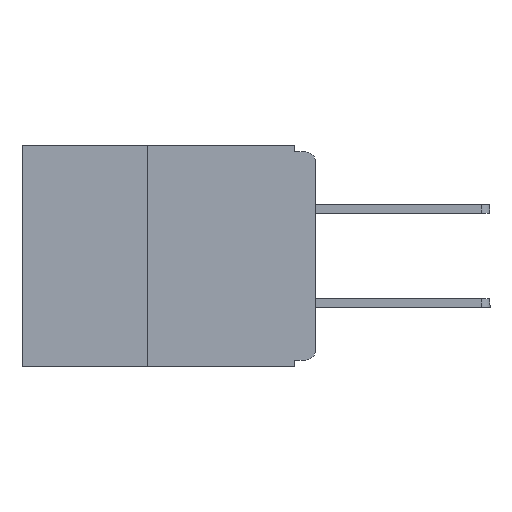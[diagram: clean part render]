
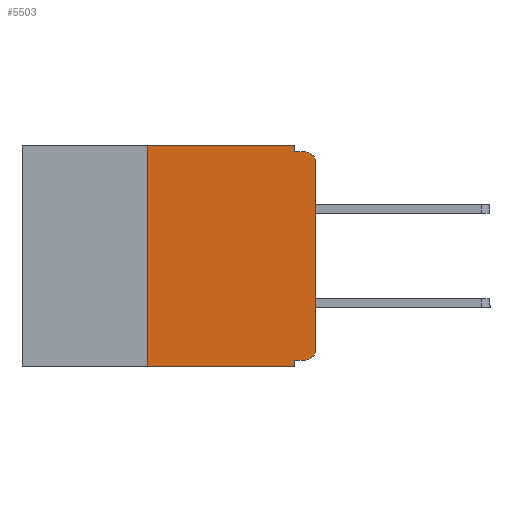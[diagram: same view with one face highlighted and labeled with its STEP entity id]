
A CAD part, left-side view. The second image highlights one B-rep face of the part: STEP entity #5503.
In plain terms, the highlighted planar face has unit normal (-1, 0, 0).
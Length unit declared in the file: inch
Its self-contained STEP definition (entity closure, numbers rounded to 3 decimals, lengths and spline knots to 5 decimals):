
#1129 = CARTESIAN_POINT ( 'NONE',  ( 0., 0.015, -0.01 ) ) ;
#1222 = CARTESIAN_POINT ( 'NONE',  ( 0., 0.25, 0. ) ) ;
#1565 = AXIS2_PLACEMENT_3D ( 'NONE', #5508, #13372, #6719 ) ;
#1937 = DIRECTION ( 'NONE',  ( 0., 0., 1. ) ) ;
#1966 = DIRECTION ( 'NONE',  ( 0., 0., -1. ) ) ;
#1986 = DIRECTION ( 'NONE',  ( 1., 0., 0. ) ) ;
#2007 = PLANE ( 'NONE',  #13067 ) ;
#2136 = CARTESIAN_POINT ( 'NONE',  ( 0., 0., -0.01 ) ) ;
#2154 = CARTESIAN_POINT ( 'NONE',  ( 0., 0.437, 0. ) ) ;
#2473 = FACE_OUTER_BOUND ( 'NONE', #12081, .T. ) ;
#2479 = VECTOR ( 'NONE', #6646, 39.37008 ) ;
#2536 = ORIENTED_EDGE ( 'NONE', *, *, #13126, .T. ) ;
#2957 = CARTESIAN_POINT ( 'NONE',  ( 0., 0., 0. ) ) ;
#3053 = LINE ( 'NONE', #10848, #14313 ) ;
#3094 = ORIENTED_EDGE ( 'NONE', *, *, #9424, .T. ) ;
#3125 = ORIENTED_EDGE ( 'NONE', *, *, #6260, .F. ) ;
#3194 = EDGE_CURVE ( 'NONE', #7947, #13280, #8759, .T. ) ;
#3290 = DIRECTION ( 'NONE',  ( 0., -1., 0. ) ) ;
#3303 = ORIENTED_EDGE ( 'NONE', *, *, #8119, .T. ) ;
#3767 = CARTESIAN_POINT ( 'NONE',  ( 0., 0.25, -0.33 ) ) ;
#4493 = VERTEX_POINT ( 'NONE', #13315 ) ;
#4528 = LINE ( 'NONE', #5465, #4894 ) ;
#4581 = VERTEX_POINT ( 'NONE', #12604 ) ;
#4690 = ORIENTED_EDGE ( 'NONE', *, *, #8791, .F. ) ;
#4702 = VECTOR ( 'NONE', #6702, 39.37008 ) ;
#4733 = ORIENTED_EDGE ( 'NONE', *, *, #3194, .F. ) ;
#4763 = CARTESIAN_POINT ( 'NONE',  ( 0., 0.031, 0. ) ) ;
#4802 = CARTESIAN_POINT ( 'NONE',  ( 0., 0., -0.025 ) ) ;
#4886 = VERTEX_POINT ( 'NONE', #9381 ) ;
#4894 = VECTOR ( 'NONE', #14404, 39.37008 ) ;
#5351 = VERTEX_POINT ( 'NONE', #4802 ) ;
#5465 = CARTESIAN_POINT ( 'NONE',  ( 0., 0.437, 0. ) ) ;
#5503 = ADVANCED_FACE ( 'NONE', ( #2473 ), #2007, .F. ) ;
#5508 = CARTESIAN_POINT ( 'NONE',  ( 0., 0.015, -0.305 ) ) ;
#5520 = LINE ( 'NONE', #13312, #2479 ) ;
#5572 = ORIENTED_EDGE ( 'NONE', *, *, #12054, .F. ) ;
#5578 = VECTOR ( 'NONE', #1937, 39.37008 ) ;
#5779 = VERTEX_POINT ( 'NONE', #1129 ) ;
#6260 = EDGE_CURVE ( 'NONE', #4581, #7574, #5520, .T. ) ;
#6646 = DIRECTION ( 'NONE',  ( 0., 0., -1. ) ) ;
#6651 = CARTESIAN_POINT ( 'NONE',  ( 0., 0.015, -0.025 ) ) ;
#6702 = DIRECTION ( 'NONE',  ( 0., -1., 0. ) ) ;
#6719 = DIRECTION ( 'NONE',  ( 0., 0., -1. ) ) ;
#7454 = EDGE_CURVE ( 'NONE', #4493, #5351, #14241, .T. ) ;
#7574 = VERTEX_POINT ( 'NONE', #11229 ) ;
#7851 = LINE ( 'NONE', #11214, #4702 ) ;
#7855 = DIRECTION ( 'NONE',  ( 0., 0., -1. ) ) ;
#7947 = VERTEX_POINT ( 'NONE', #3767 ) ;
#8119 = EDGE_CURVE ( 'NONE', #5351, #5779, #13058, .T. ) ;
#8693 = CARTESIAN_POINT ( 'NONE',  ( 0., 0.031, -0.01 ) ) ;
#8759 = LINE ( 'NONE', #14010, #5578 ) ;
#8783 = CIRCLE ( 'NONE', #1565, 0.015 ) ;
#8791 = EDGE_CURVE ( 'NONE', #13280, #14341, #4528, .T. ) ;
#8995 = LINE ( 'NONE', #2136, #14379 ) ;
#9381 = CARTESIAN_POINT ( 'NONE',  ( 0., 0.015, -0.32 ) ) ;
#9424 = EDGE_CURVE ( 'NONE', #7947, #7574, #7851, .T. ) ;
#9477 = DIRECTION ( 'NONE',  ( 0., 0., -1. ) ) ;
#10304 = EDGE_CURVE ( 'NONE', #14341, #10970, #13990, .T. ) ;
#10848 = CARTESIAN_POINT ( 'NONE',  ( 0., 0., -0.32 ) ) ;
#10970 = VERTEX_POINT ( 'NONE', #8693 ) ;
#11214 = CARTESIAN_POINT ( 'NONE',  ( 0., 0.437, -0.33 ) ) ;
#11229 = CARTESIAN_POINT ( 'NONE',  ( 0., 0.031, -0.33 ) ) ;
#11379 = AXIS2_PLACEMENT_3D ( 'NONE', #6651, #14397, #7855 ) ;
#11402 = VECTOR ( 'NONE', #12088, 39.37008 ) ;
#11905 = DIRECTION ( 'NONE',  ( 0., 1., 0. ) ) ;
#12054 = EDGE_CURVE ( 'NONE', #10970, #5779, #8995, .T. ) ;
#12081 = EDGE_LOOP ( 'NONE', ( #13181, #3303, #5572, #13323, #4690, #4733, #3094, #3125, #12618, #2536 ) ) ;
#12088 = DIRECTION ( 'NONE',  ( 0., 0., 1. ) ) ;
#12564 = CARTESIAN_POINT ( 'NONE',  ( 0., 0.031, 0. ) ) ;
#12604 = CARTESIAN_POINT ( 'NONE',  ( 0., 0.031, -0.32 ) ) ;
#12618 = ORIENTED_EDGE ( 'NONE', *, *, #14145, .F. ) ;
#13058 = CIRCLE ( 'NONE', #11379, 0.015 ) ;
#13067 = AXIS2_PLACEMENT_3D ( 'NONE', #2154, #1986, #1966 ) ;
#13126 = EDGE_CURVE ( 'NONE', #4886, #4493, #8783, .T. ) ;
#13181 = ORIENTED_EDGE ( 'NONE', *, *, #7454, .T. ) ;
#13280 = VERTEX_POINT ( 'NONE', #1222 ) ;
#13312 = CARTESIAN_POINT ( 'NONE',  ( 0., 0.031, -0.33 ) ) ;
#13315 = CARTESIAN_POINT ( 'NONE',  ( 0., 0., -0.305 ) ) ;
#13323 = ORIENTED_EDGE ( 'NONE', *, *, #10304, .F. ) ;
#13372 = DIRECTION ( 'NONE',  ( -1., 0., 0. ) ) ;
#13660 = VECTOR ( 'NONE', #9477, 39.37008 ) ;
#13990 = LINE ( 'NONE', #4763, #13660 ) ;
#14010 = CARTESIAN_POINT ( 'NONE',  ( 0., 0.25, -0.33 ) ) ;
#14145 = EDGE_CURVE ( 'NONE', #4886, #4581, #3053, .T. ) ;
#14241 = LINE ( 'NONE', #2957, #11402 ) ;
#14313 = VECTOR ( 'NONE', #11905, 39.37008 ) ;
#14341 = VERTEX_POINT ( 'NONE', #12564 ) ;
#14379 = VECTOR ( 'NONE', #3290, 39.37008 ) ;
#14397 = DIRECTION ( 'NONE',  ( -1., 0., 0. ) ) ;
#14404 = DIRECTION ( 'NONE',  ( 0., -1., 0. ) ) ;
